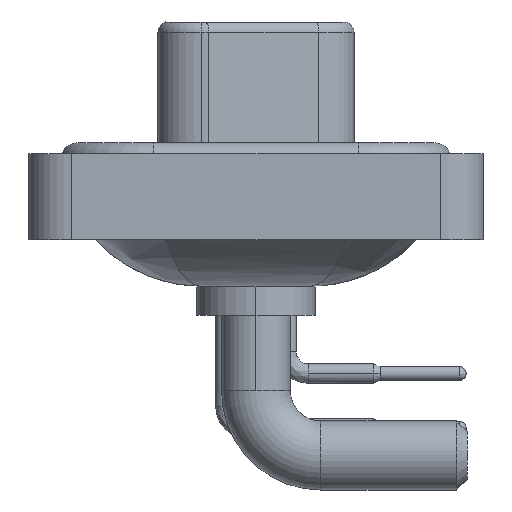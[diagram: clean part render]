
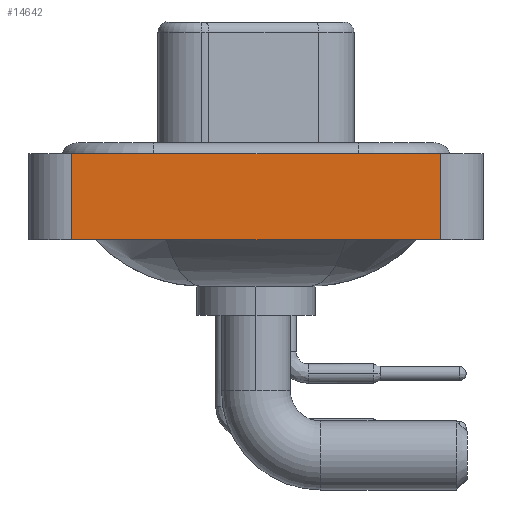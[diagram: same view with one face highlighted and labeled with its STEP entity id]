
A CAD part, left-side view. The second image highlights one B-rep face of the part: STEP entity #14642.
In plain terms, the highlighted planar face has unit normal (-1, 0, 0).
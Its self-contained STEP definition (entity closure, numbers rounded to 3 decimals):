
#162 = EDGE_CURVE ( 'NONE', #20374, #3652, #5234, .T. ) ;
#525 = VECTOR ( 'NONE', #18134, 1000. ) ;
#2880 = EDGE_LOOP ( 'NONE', ( #5912, #5670, #16132, #21233 ) ) ;
#3453 = PLANE ( 'NONE',  #17970 ) ;
#3592 = DIRECTION ( 'NONE',  ( 0., 0., 1. ) ) ;
#3652 = VERTEX_POINT ( 'NONE', #11953 ) ;
#3887 = VECTOR ( 'NONE', #16349, 1000. ) ;
#4512 = EDGE_CURVE ( 'NONE', #15003, #3652, #16606, .T. ) ;
#5234 = LINE ( 'NONE', #18874, #13397 ) ;
#5616 = CARTESIAN_POINT ( 'NONE',  ( -7.3, 8.55, 0.4 ) ) ;
#5670 = ORIENTED_EDGE ( 'NONE', *, *, #162, .F. ) ;
#5912 = ORIENTED_EDGE ( 'NONE', *, *, #4512, .T. ) ;
#6558 = LINE ( 'NONE', #12137, #3887 ) ;
#9291 = CARTESIAN_POINT ( 'NONE',  ( -7.3, -8.55, -3.6 ) ) ;
#10912 = DIRECTION ( 'NONE',  ( -1., 0., 0. ) ) ;
#11166 = EDGE_CURVE ( 'NONE', #16270, #15003, #14270, .T. ) ;
#11953 = CARTESIAN_POINT ( 'NONE',  ( -7.3, -8.55, 0.4 ) ) ;
#12137 = CARTESIAN_POINT ( 'NONE',  ( -7.3, 8.55, -3.6 ) ) ;
#12758 = VECTOR ( 'NONE', #3592, 1000. ) ;
#13397 = VECTOR ( 'NONE', #16637, 1000. ) ;
#14270 = LINE ( 'NONE', #23835, #525 ) ;
#14642 = ADVANCED_FACE ( 'NONE', ( #20831 ), #3453, .T. ) ;
#15003 = VERTEX_POINT ( 'NONE', #18325 ) ;
#16132 = ORIENTED_EDGE ( 'NONE', *, *, #22676, .F. ) ;
#16270 = VERTEX_POINT ( 'NONE', #16952 ) ;
#16349 = DIRECTION ( 'NONE',  ( 0., 0., 1. ) ) ;
#16606 = LINE ( 'NONE', #24174, #12758 ) ;
#16637 = DIRECTION ( 'NONE',  ( 0., -1., 0. ) ) ;
#16952 = CARTESIAN_POINT ( 'NONE',  ( -7.3, 8.55, -3.6 ) ) ;
#17970 = AXIS2_PLACEMENT_3D ( 'NONE', #9291, #10912, #24399 ) ;
#18134 = DIRECTION ( 'NONE',  ( 0., -1., 0. ) ) ;
#18325 = CARTESIAN_POINT ( 'NONE',  ( -7.3, -8.55, -3.6 ) ) ;
#18874 = CARTESIAN_POINT ( 'NONE',  ( -7.3, -8.55, 0.4 ) ) ;
#20374 = VERTEX_POINT ( 'NONE', #5616 ) ;
#20831 = FACE_OUTER_BOUND ( 'NONE', #2880, .T. ) ;
#21233 = ORIENTED_EDGE ( 'NONE', *, *, #11166, .T. ) ;
#22676 = EDGE_CURVE ( 'NONE', #16270, #20374, #6558, .T. ) ;
#23835 = CARTESIAN_POINT ( 'NONE',  ( -7.3, -8.55, -3.6 ) ) ;
#24174 = CARTESIAN_POINT ( 'NONE',  ( -7.3, -8.55, -3.6 ) ) ;
#24399 = DIRECTION ( 'NONE',  ( 0., 0., 1. ) ) ;
